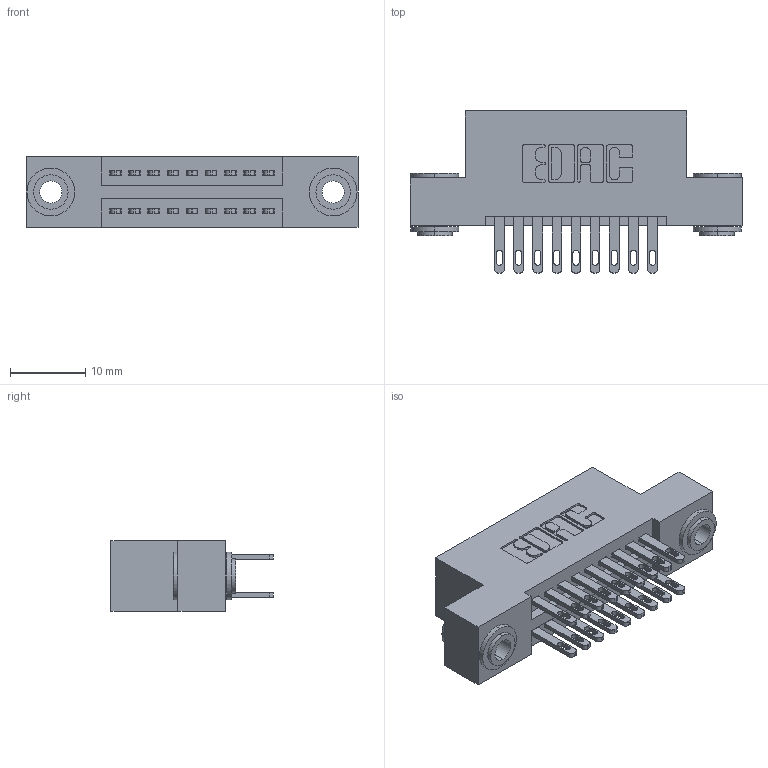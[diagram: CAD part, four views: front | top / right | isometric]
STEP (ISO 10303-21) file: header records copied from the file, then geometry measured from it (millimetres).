
FILE_DESCRIPTION (( 'STEP AP203' ), '1' );
FILE_NAME ('895-018-500-203.STEP', '2020-09-25T05:59:19', ( '' ), ( '' ), 'SwSTEP 2.0', 'SolidWorks 2020', '' );
FILE_SCHEMA (( 'CONFIG_CONTROL_DESIGN' ));
Length unit declared in the file: inch
Products named in the file (4): 895-018-500-203; 345-292-001_345-293-100; 845 Part_Flush Mounting Lugs - 0.156 Dia-TH; 345-250-002_345-250-002-102
Assembly tree (21 placements, depth 2):
  895-018-500-203
    845 Part_Flush Mounting Lugs - 0.156 Dia-TH
    345-292-001_345-293-100  x18
    345-250-002_345-250-002-102  x2
Bounding box: 44.07 x 21.51 x 9.4 mm (x, y, z)
Volume: 4049 mm3; surface area: 5734.4 mm2
Topology: 21 solids, 21 shells, 992 faces, 2955 edges, 1966 vertices
Faces by surface type: plane 576, cylinder 408, cone 8
Entity records: 12084 total; most frequent: CARTESIAN_POINT 2031, ORIENTED_EDGE 1958, DIRECTION 1865, EDGE_CURVE 979, VECTOR 783, LINE 783, VERTEX_POINT 650, AXIS2_PLACEMENT_3D 541
